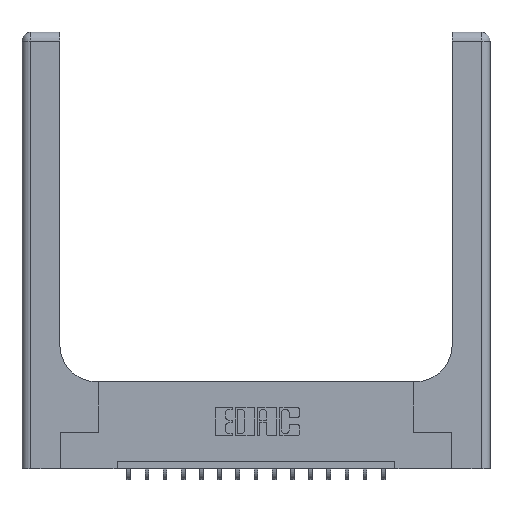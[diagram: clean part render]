
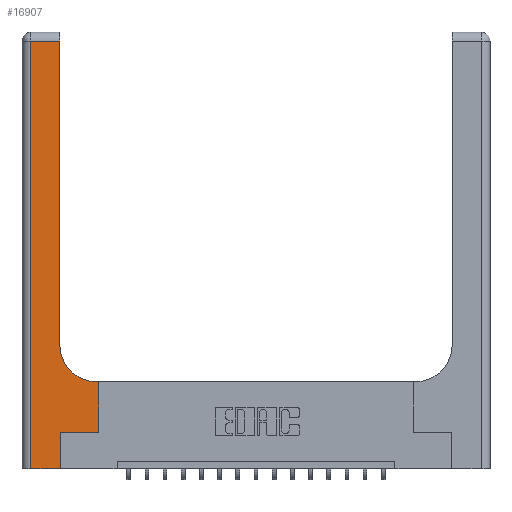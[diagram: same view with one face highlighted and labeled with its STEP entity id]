
A CAD part, top view. The second image highlights one B-rep face of the part: STEP entity #16907.
In plain terms, the highlighted planar face has unit normal (0, 0, 1).
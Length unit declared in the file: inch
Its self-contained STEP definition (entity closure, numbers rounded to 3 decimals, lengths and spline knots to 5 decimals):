
#6 = ORIENTED_EDGE ( 'NONE', *, *, #16820, .T. ) ;
#157 = DIRECTION ( 'NONE',  ( 1., 0., 0. ) ) ;
#281 = DIRECTION ( 'NONE',  ( 0., 0., -1. ) ) ;
#851 = CARTESIAN_POINT ( 'NONE',  ( 0.06, 0., 0.37 ) ) ;
#924 = CARTESIAN_POINT ( 'NONE',  ( 0.265, 0.25, 0.37 ) ) ;
#1153 = CARTESIAN_POINT ( 'NONE',  ( 0.06, 2.94, 0.37 ) ) ;
#1180 = VECTOR ( 'NONE', #5585, 39.37008 ) ;
#1385 = EDGE_LOOP ( 'NONE', ( #16944, #2478, #10998, #13883, #6, #7969, #11916, #3001, #9812 ) ) ;
#1704 = CARTESIAN_POINT ( 'NONE',  ( 0.265, 0., 0.37 ) ) ;
#1807 = VERTEX_POINT ( 'NONE', #1153 ) ;
#2081 = CARTESIAN_POINT ( 'NONE',  ( 0.26, 3., 0.37 ) ) ;
#2478 = ORIENTED_EDGE ( 'NONE', *, *, #14407, .T. ) ;
#2625 = VERTEX_POINT ( 'NONE', #9970 ) ;
#2843 = VECTOR ( 'NONE', #157, 39.37008 ) ;
#2918 = FACE_OUTER_BOUND ( 'NONE', #1385, .T. ) ;
#3001 = ORIENTED_EDGE ( 'NONE', *, *, #11480, .T. ) ;
#3264 = LINE ( 'NONE', #17096, #2843 ) ;
#3305 = EDGE_CURVE ( 'NONE', #2625, #9476, #16526, .T. ) ;
#3483 = DIRECTION ( 'NONE',  ( 1., 0., 0. ) ) ;
#3856 = VECTOR ( 'NONE', #12286, 39.37008 ) ;
#4289 = LINE ( 'NONE', #15076, #3856 ) ;
#4571 = CIRCLE ( 'NONE', #5039, 0.25 ) ;
#4645 = PLANE ( 'NONE',  #8219 ) ;
#4742 = CARTESIAN_POINT ( 'NONE',  ( 0.26, 0.6, 0.37 ) ) ;
#5013 = EDGE_CURVE ( 'NONE', #14859, #2625, #3264, .T. ) ;
#5039 = AXIS2_PLACEMENT_3D ( 'NONE', #8763, #281, #10182 ) ;
#5213 = CARTESIAN_POINT ( 'NONE',  ( 0.26, 2.94, 0.37 ) ) ;
#5585 = DIRECTION ( 'NONE',  ( -1., 0., 0. ) ) ;
#6080 = DIRECTION ( 'NONE',  ( 0., 0., -1. ) ) ;
#6235 = VERTEX_POINT ( 'NONE', #17358 ) ;
#6874 = VERTEX_POINT ( 'NONE', #10745 ) ;
#7717 = CARTESIAN_POINT ( 'NONE',  ( 0., 0., 0.37 ) ) ;
#7912 = VECTOR ( 'NONE', #14788, 39.37008 ) ;
#7968 = VECTOR ( 'NONE', #10096, 39.37008 ) ;
#7969 = ORIENTED_EDGE ( 'NONE', *, *, #5013, .T. ) ;
#8219 = AXIS2_PLACEMENT_3D ( 'NONE', #14523, #6080, #15921 ) ;
#8521 = EDGE_CURVE ( 'NONE', #11681, #6235, #12976, .T. ) ;
#8763 = CARTESIAN_POINT ( 'NONE',  ( 0.51, 0.85, 0.37 ) ) ;
#9016 = EDGE_CURVE ( 'NONE', #9592, #6874, #4571, .T. ) ;
#9476 = VERTEX_POINT ( 'NONE', #11199 ) ;
#9592 = VERTEX_POINT ( 'NONE', #15812 ) ;
#9812 = ORIENTED_EDGE ( 'NONE', *, *, #9016, .T. ) ;
#9851 = CARTESIAN_POINT ( 'NONE',  ( 0., 2.94, 0.37 ) ) ;
#9970 = CARTESIAN_POINT ( 'NONE',  ( 0.528, 0.25, 0.37 ) ) ;
#10096 = DIRECTION ( 'NONE',  ( 0., 1., 0. ) ) ;
#10182 = DIRECTION ( 'NONE',  ( 1., 0., 0. ) ) ;
#10224 = LINE ( 'NONE', #4742, #17642 ) ;
#10745 = CARTESIAN_POINT ( 'NONE',  ( 0.26, 0.85, 0.37 ) ) ;
#10794 = VERTEX_POINT ( 'NONE', #5213 ) ;
#10998 = ORIENTED_EDGE ( 'NONE', *, *, #14896, .T. ) ;
#11199 = CARTESIAN_POINT ( 'NONE',  ( 0.528, 0.6, 0.37 ) ) ;
#11480 = EDGE_CURVE ( 'NONE', #9476, #9592, #10224, .T. ) ;
#11651 = LINE ( 'NONE', #2081, #7912 ) ;
#11681 = VERTEX_POINT ( 'NONE', #851 ) ;
#11916 = ORIENTED_EDGE ( 'NONE', *, *, #3305, .T. ) ;
#12088 = VECTOR ( 'NONE', #3483, 39.37008 ) ;
#12286 = DIRECTION ( 'NONE',  ( 0., -1., 0. ) ) ;
#12805 = VECTOR ( 'NONE', #14320, 39.37008 ) ;
#12884 = CARTESIAN_POINT ( 'NONE',  ( 0.528, 0.25, 0.37 ) ) ;
#12976 = LINE ( 'NONE', #7717, #12088 ) ;
#13883 = ORIENTED_EDGE ( 'NONE', *, *, #8521, .T. ) ;
#14320 = DIRECTION ( 'NONE',  ( 0., 1., 0. ) ) ;
#14407 = EDGE_CURVE ( 'NONE', #10794, #1807, #15743, .T. ) ;
#14523 = CARTESIAN_POINT ( 'NONE',  ( 0., 3., 0.37 ) ) ;
#14628 = DIRECTION ( 'NONE',  ( -1., 0., 0. ) ) ;
#14788 = DIRECTION ( 'NONE',  ( 0., 1., 0. ) ) ;
#14859 = VERTEX_POINT ( 'NONE', #924 ) ;
#14896 = EDGE_CURVE ( 'NONE', #1807, #11681, #4289, .T. ) ;
#15047 = LINE ( 'NONE', #1704, #7968 ) ;
#15076 = CARTESIAN_POINT ( 'NONE',  ( 0.06, 3., 0.37 ) ) ;
#15743 = LINE ( 'NONE', #9851, #1180 ) ;
#15812 = CARTESIAN_POINT ( 'NONE',  ( 0.51, 0.6, 0.37 ) ) ;
#15921 = DIRECTION ( 'NONE',  ( -1., 0., 0. ) ) ;
#16526 = LINE ( 'NONE', #12884, #12805 ) ;
#16820 = EDGE_CURVE ( 'NONE', #6235, #14859, #15047, .T. ) ;
#16907 = ADVANCED_FACE ( 'NONE', ( #2918 ), #4645, .F. ) ;
#16944 = ORIENTED_EDGE ( 'NONE', *, *, #18109, .T. ) ;
#17096 = CARTESIAN_POINT ( 'NONE',  ( 0.265, 0.25, 0.37 ) ) ;
#17358 = CARTESIAN_POINT ( 'NONE',  ( 0.265, 0., 0.37 ) ) ;
#17642 = VECTOR ( 'NONE', #14628, 39.37008 ) ;
#18109 = EDGE_CURVE ( 'NONE', #6874, #10794, #11651, .T. ) ;
